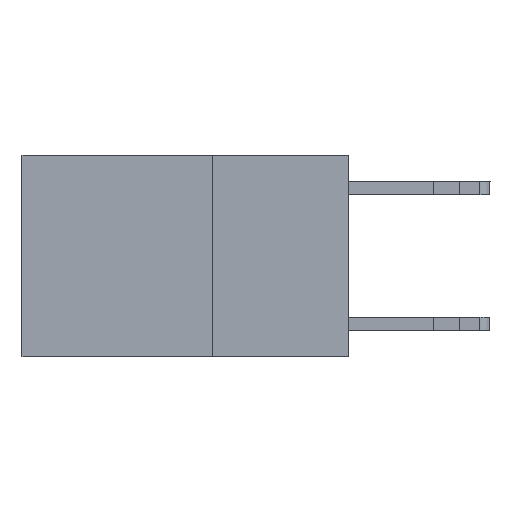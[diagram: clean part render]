
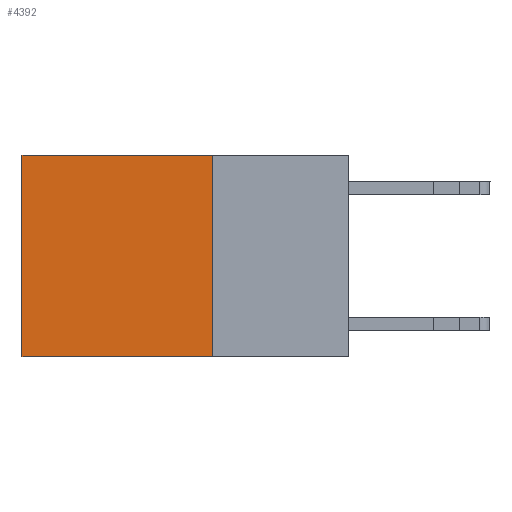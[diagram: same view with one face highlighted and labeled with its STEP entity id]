
A CAD part, left-side view. The second image highlights one B-rep face of the part: STEP entity #4392.
In plain terms, the highlighted planar face has unit normal (-1, 0, 0).
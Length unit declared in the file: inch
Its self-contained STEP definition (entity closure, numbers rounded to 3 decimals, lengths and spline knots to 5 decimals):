
#809 = LINE ( 'NONE', #21957, #16591 ) ;
#1426 = EDGE_LOOP ( 'NONE', ( #6481, #20370, #7428, #15787 ) ) ;
#1929 = CARTESIAN_POINT ( 'NONE',  ( 0.2625, 0.25, 0. ) ) ;
#2498 = EDGE_CURVE ( 'NONE', #9006, #10441, #11932, .T. ) ;
#2790 = CARTESIAN_POINT ( 'NONE',  ( 0.2625, 0.6, 0. ) ) ;
#2811 = CARTESIAN_POINT ( 'NONE',  ( 0.2625, 0.6, -0.37 ) ) ;
#4392 = ADVANCED_FACE ( 'NONE', ( #15635 ), #19640, .F. ) ;
#4650 = VECTOR ( 'NONE', #20131, 39.37008 ) ;
#4791 = VECTOR ( 'NONE', #17080, 39.37008 ) ;
#5667 = DIRECTION ( 'NONE',  ( 1., 0., 0. ) ) ;
#6481 = ORIENTED_EDGE ( 'NONE', *, *, #2498, .T. ) ;
#6707 = CARTESIAN_POINT ( 'NONE',  ( 0.2625, 0.25, 0. ) ) ;
#7123 = EDGE_CURVE ( 'NONE', #14615, #10441, #21857, .T. ) ;
#7428 = ORIENTED_EDGE ( 'NONE', *, *, #11364, .F. ) ;
#7608 = AXIS2_PLACEMENT_3D ( 'NONE', #1929, #5667, #19195 ) ;
#8376 = LINE ( 'NONE', #15123, #19553 ) ;
#9006 = VERTEX_POINT ( 'NONE', #2790 ) ;
#10102 = CARTESIAN_POINT ( 'NONE',  ( 0.2625, 0.6, 0. ) ) ;
#10441 = VERTEX_POINT ( 'NONE', #2811 ) ;
#11364 = EDGE_CURVE ( 'NONE', #13659, #14615, #809, .T. ) ;
#11932 = LINE ( 'NONE', #10102, #4791 ) ;
#13659 = VERTEX_POINT ( 'NONE', #6707 ) ;
#14615 = VERTEX_POINT ( 'NONE', #21276 ) ;
#14633 = CARTESIAN_POINT ( 'NONE',  ( 0.2625, 0.25, -0.37 ) ) ;
#15123 = CARTESIAN_POINT ( 'NONE',  ( 0.2625, 0.25, 0. ) ) ;
#15201 = EDGE_CURVE ( 'NONE', #13659, #9006, #8376, .T. ) ;
#15635 = FACE_OUTER_BOUND ( 'NONE', #1426, .T. ) ;
#15787 = ORIENTED_EDGE ( 'NONE', *, *, #15201, .T. ) ;
#16591 = VECTOR ( 'NONE', #22071, 39.37008 ) ;
#17080 = DIRECTION ( 'NONE',  ( 0., 0., -1. ) ) ;
#19195 = DIRECTION ( 'NONE',  ( 0., 0., -1. ) ) ;
#19553 = VECTOR ( 'NONE', #20405, 39.37008 ) ;
#19640 = PLANE ( 'NONE',  #7608 ) ;
#20131 = DIRECTION ( 'NONE',  ( 0., 1., 0. ) ) ;
#20370 = ORIENTED_EDGE ( 'NONE', *, *, #7123, .F. ) ;
#20405 = DIRECTION ( 'NONE',  ( 0., 1., 0. ) ) ;
#21276 = CARTESIAN_POINT ( 'NONE',  ( 0.2625, 0.25, -0.37 ) ) ;
#21857 = LINE ( 'NONE', #14633, #4650 ) ;
#21957 = CARTESIAN_POINT ( 'NONE',  ( 0.2625, 0.25, 0. ) ) ;
#22071 = DIRECTION ( 'NONE',  ( 0., 0., -1. ) ) ;
